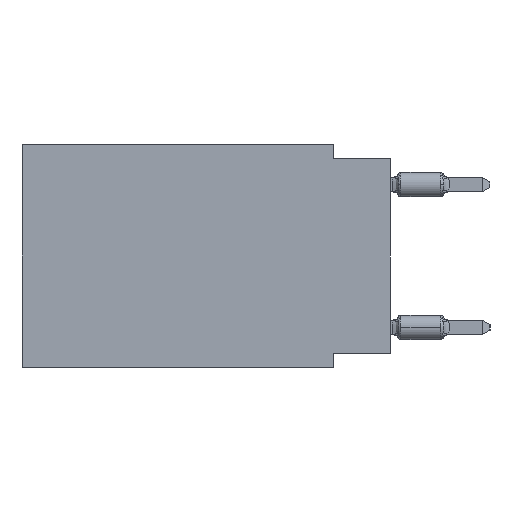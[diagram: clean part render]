
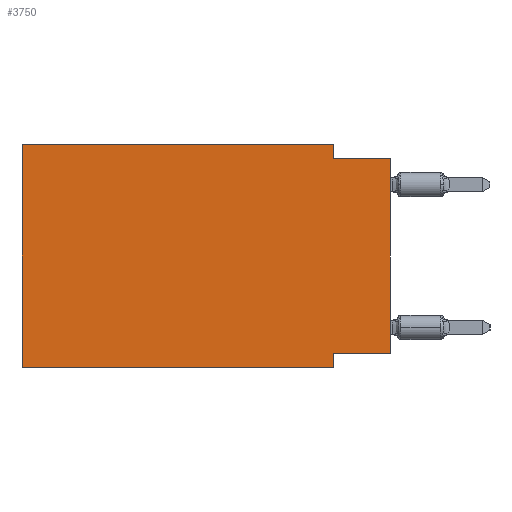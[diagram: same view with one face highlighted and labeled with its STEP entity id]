
A CAD part, left-side view. The second image highlights one B-rep face of the part: STEP entity #3750.
In plain terms, the highlighted planar face has unit normal (-1, 0, 0).
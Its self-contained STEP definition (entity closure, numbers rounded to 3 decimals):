
#307 = CARTESIAN_POINT ( 'NONE',  ( 0., 2.54, 0. ) ) ;
#362 = DIRECTION ( 'NONE',  ( 1., 0., 0. ) ) ;
#524 = ORIENTED_EDGE ( 'NONE', *, *, #13051, .T. ) ;
#800 = EDGE_CURVE ( 'NONE', #50917, #4708, #50101, .T. ) ;
#1877 = VECTOR ( 'NONE', #26839, 1000. ) ;
#1883 = VECTOR ( 'NONE', #38407, 1000. ) ;
#2342 = DIRECTION ( 'NONE',  ( 0., 0., 1. ) ) ;
#2785 = EDGE_CURVE ( 'NONE', #31283, #4708, #57538, .T. ) ;
#2824 = VERTEX_POINT ( 'NONE', #25677 ) ;
#3619 = CARTESIAN_POINT ( 'NONE',  ( 0., 2.54, -0.635 ) ) ;
#3750 = ADVANCED_FACE ( 'NONE', ( #36065 ), #49511, .F. ) ;
#4590 = ORIENTED_EDGE ( 'NONE', *, *, #39138, .F. ) ;
#4708 = VERTEX_POINT ( 'NONE', #38427 ) ;
#6042 = VERTEX_POINT ( 'NONE', #54006 ) ;
#6162 = LINE ( 'NONE', #10567, #7453 ) ;
#7095 = LINE ( 'NONE', #35757, #11820 ) ;
#7453 = VECTOR ( 'NONE', #2342, 1000. ) ;
#7848 = CARTESIAN_POINT ( 'NONE',  ( 0., 0., -0.635 ) ) ;
#8271 = LINE ( 'NONE', #30196, #17116 ) ;
#9838 = DIRECTION ( 'NONE',  ( 0., 0., -1. ) ) ;
#10567 = CARTESIAN_POINT ( 'NONE',  ( 0., 16.383, 0. ) ) ;
#10607 = CARTESIAN_POINT ( 'NONE',  ( 0., 0., 0. ) ) ;
#11820 = VECTOR ( 'NONE', #13820, 1000. ) ;
#12235 = VERTEX_POINT ( 'NONE', #44975 ) ;
#12505 = EDGE_CURVE ( 'NONE', #38291, #31283, #7095, .T. ) ;
#13051 = EDGE_CURVE ( 'NONE', #12235, #2824, #23387, .T. ) ;
#13820 = DIRECTION ( 'NONE',  ( 0., 0., -1. ) ) ;
#13831 = CARTESIAN_POINT ( 'NONE',  ( 0., 16.383, 0. ) ) ;
#16490 = EDGE_CURVE ( 'NONE', #12235, #54392, #6162, .T. ) ;
#17116 = VECTOR ( 'NONE', #38391, 1000. ) ;
#17217 = EDGE_CURVE ( 'NONE', #54392, #38291, #24365, .T. ) ;
#17667 = ORIENTED_EDGE ( 'NONE', *, *, #20310, .F. ) ;
#18331 = LINE ( 'NONE', #18900, #54013 ) ;
#18900 = CARTESIAN_POINT ( 'NONE',  ( 0., 2.54, -9.906 ) ) ;
#19566 = CARTESIAN_POINT ( 'NONE',  ( 0., 16.383, -9.906 ) ) ;
#20310 = EDGE_CURVE ( 'NONE', #50917, #6042, #8271, .T. ) ;
#20916 = CARTESIAN_POINT ( 'NONE',  ( 0., 16.383, 0. ) ) ;
#21741 = ORIENTED_EDGE ( 'NONE', *, *, #12505, .F. ) ;
#23387 = LINE ( 'NONE', #19566, #39954 ) ;
#24226 = DIRECTION ( 'NONE',  ( 0., -1., 0. ) ) ;
#24365 = LINE ( 'NONE', #28764, #1883 ) ;
#25677 = CARTESIAN_POINT ( 'NONE',  ( 0., 2.54, -9.906 ) ) ;
#26839 = DIRECTION ( 'NONE',  ( 0., -1., 0. ) ) ;
#27775 = VECTOR ( 'NONE', #28447, 1000. ) ;
#28447 = DIRECTION ( 'NONE',  ( 0., 0., 1. ) ) ;
#28764 = CARTESIAN_POINT ( 'NONE',  ( 0., 16.383, 0. ) ) ;
#29435 = ORIENTED_EDGE ( 'NONE', *, *, #16490, .F. ) ;
#30196 = CARTESIAN_POINT ( 'NONE',  ( 0., 0., -9.271 ) ) ;
#30235 = ORIENTED_EDGE ( 'NONE', *, *, #17217, .F. ) ;
#31027 = ORIENTED_EDGE ( 'NONE', *, *, #800, .T. ) ;
#31283 = VERTEX_POINT ( 'NONE', #3619 ) ;
#35757 = CARTESIAN_POINT ( 'NONE',  ( 0., 2.54, 0. ) ) ;
#36065 = FACE_OUTER_BOUND ( 'NONE', #40226, .T. ) ;
#38291 = VERTEX_POINT ( 'NONE', #307 ) ;
#38391 = DIRECTION ( 'NONE',  ( 0., 1., 0. ) ) ;
#38407 = DIRECTION ( 'NONE',  ( 0., -1., 0. ) ) ;
#38427 = CARTESIAN_POINT ( 'NONE',  ( 0., 0., -0.635 ) ) ;
#39138 = EDGE_CURVE ( 'NONE', #6042, #2824, #18331, .T. ) ;
#39954 = VECTOR ( 'NONE', #24226, 1000. ) ;
#40226 = EDGE_LOOP ( 'NONE', ( #31027, #56667, #21741, #30235, #29435, #524, #4590, #17667 ) ) ;
#43942 = CARTESIAN_POINT ( 'NONE',  ( 0., 0., -9.271 ) ) ;
#44975 = CARTESIAN_POINT ( 'NONE',  ( 0., 16.383, -9.906 ) ) ;
#45932 = AXIS2_PLACEMENT_3D ( 'NONE', #13831, #362, #54464 ) ;
#49511 = PLANE ( 'NONE',  #45932 ) ;
#50101 = LINE ( 'NONE', #10607, #27775 ) ;
#50917 = VERTEX_POINT ( 'NONE', #43942 ) ;
#54006 = CARTESIAN_POINT ( 'NONE',  ( 0., 2.54, -9.271 ) ) ;
#54013 = VECTOR ( 'NONE', #9838, 1000. ) ;
#54392 = VERTEX_POINT ( 'NONE', #20916 ) ;
#54464 = DIRECTION ( 'NONE',  ( 0., 0., -1. ) ) ;
#56667 = ORIENTED_EDGE ( 'NONE', *, *, #2785, .F. ) ;
#57538 = LINE ( 'NONE', #7848, #1877 ) ;
